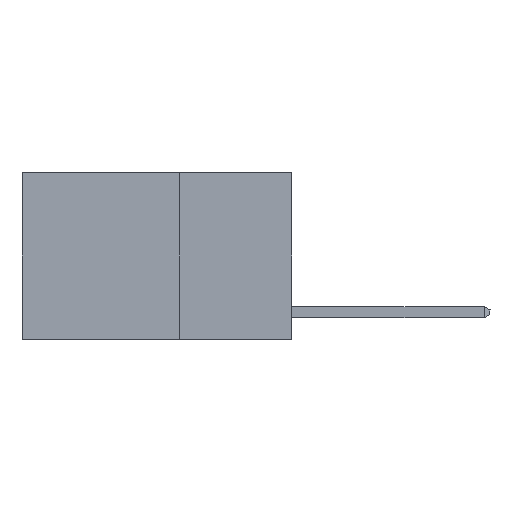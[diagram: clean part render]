
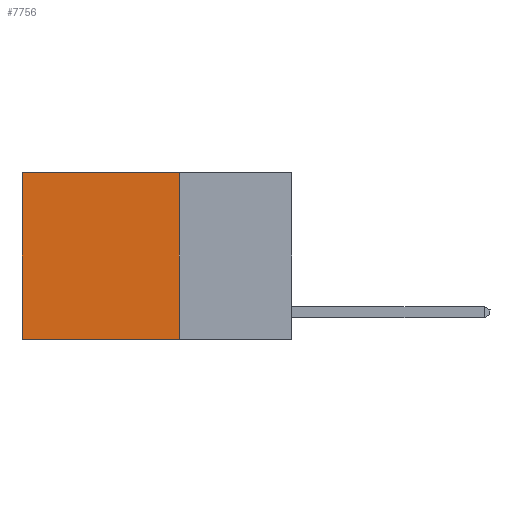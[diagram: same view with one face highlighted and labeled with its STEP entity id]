
A CAD part, left-side view. The second image highlights one B-rep face of the part: STEP entity #7756.
In plain terms, the highlighted planar face has unit normal (-1, 0, 0).
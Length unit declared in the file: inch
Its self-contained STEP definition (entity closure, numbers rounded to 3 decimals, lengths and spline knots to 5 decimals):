
#48 = EDGE_CURVE ( 'NONE', #8883, #3082, #13025, .T. ) ;
#65 = ORIENTED_EDGE ( 'NONE', *, *, #2059, .F. ) ;
#1572 = VECTOR ( 'NONE', #8126, 39.37008 ) ;
#1603 = DIRECTION ( 'NONE',  ( 1., 0., 0. ) ) ;
#1695 = CARTESIAN_POINT ( 'NONE',  ( 0.2625, 0.25, -0.37 ) ) ;
#1885 = LINE ( 'NONE', #3918, #4385 ) ;
#2059 = EDGE_CURVE ( 'NONE', #4107, #4063, #1885, .T. ) ;
#2072 = AXIS2_PLACEMENT_3D ( 'NONE', #11174, #1603, #9035 ) ;
#2482 = VECTOR ( 'NONE', #5226, 39.37008 ) ;
#2790 = DIRECTION ( 'NONE',  ( 0., 1., 0. ) ) ;
#3082 = VERTEX_POINT ( 'NONE', #13791 ) ;
#3637 = EDGE_CURVE ( 'NONE', #3082, #4063, #6647, .T. ) ;
#3918 = CARTESIAN_POINT ( 'NONE',  ( 0.2625, 0.25, -0.37 ) ) ;
#4063 = VERTEX_POINT ( 'NONE', #12321 ) ;
#4107 = VERTEX_POINT ( 'NONE', #1695 ) ;
#4322 = CARTESIAN_POINT ( 'NONE',  ( 0.2625, 0.25, 0. ) ) ;
#4385 = VECTOR ( 'NONE', #2790, 39.37008 ) ;
#5226 = DIRECTION ( 'NONE',  ( 0., 0., -1. ) ) ;
#6320 = VECTOR ( 'NONE', #13678, 39.37008 ) ;
#6647 = LINE ( 'NONE', #8180, #6320 ) ;
#6847 = EDGE_CURVE ( 'NONE', #8883, #4107, #10293, .T. ) ;
#7077 = ORIENTED_EDGE ( 'NONE', *, *, #6847, .F. ) ;
#7370 = ORIENTED_EDGE ( 'NONE', *, *, #48, .T. ) ;
#7500 = CARTESIAN_POINT ( 'NONE',  ( 0.2625, 0.25, 0. ) ) ;
#7756 = ADVANCED_FACE ( 'NONE', ( #9577 ), #7946, .F. ) ;
#7946 = PLANE ( 'NONE',  #2072 ) ;
#8126 = DIRECTION ( 'NONE',  ( 0., 1., 0. ) ) ;
#8180 = CARTESIAN_POINT ( 'NONE',  ( 0.2625, 0.6, 0. ) ) ;
#8472 = EDGE_LOOP ( 'NONE', ( #11918, #65, #7077, #7370 ) ) ;
#8883 = VERTEX_POINT ( 'NONE', #4322 ) ;
#9035 = DIRECTION ( 'NONE',  ( 0., 0., -1. ) ) ;
#9577 = FACE_OUTER_BOUND ( 'NONE', #8472, .T. ) ;
#10293 = LINE ( 'NONE', #10517, #2482 ) ;
#10517 = CARTESIAN_POINT ( 'NONE',  ( 0.2625, 0.25, 0. ) ) ;
#11174 = CARTESIAN_POINT ( 'NONE',  ( 0.2625, 0.25, 0. ) ) ;
#11918 = ORIENTED_EDGE ( 'NONE', *, *, #3637, .T. ) ;
#12321 = CARTESIAN_POINT ( 'NONE',  ( 0.2625, 0.6, -0.37 ) ) ;
#13025 = LINE ( 'NONE', #7500, #1572 ) ;
#13678 = DIRECTION ( 'NONE',  ( 0., 0., -1. ) ) ;
#13791 = CARTESIAN_POINT ( 'NONE',  ( 0.2625, 0.6, 0. ) ) ;
